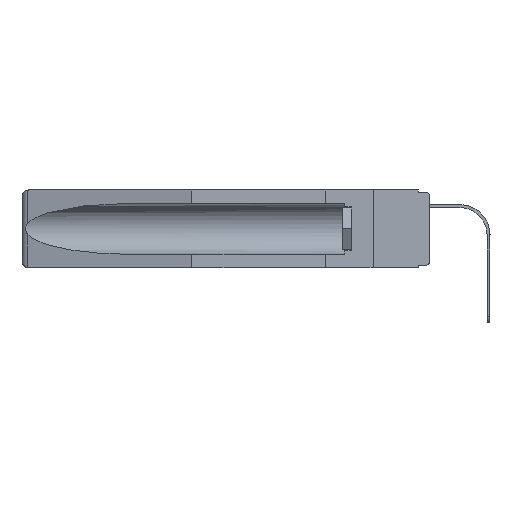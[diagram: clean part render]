
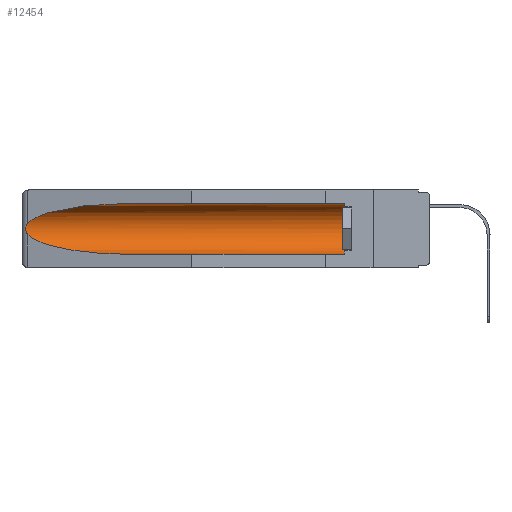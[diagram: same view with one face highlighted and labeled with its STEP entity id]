
A CAD part, left-side view. The second image highlights one B-rep face of the part: STEP entity #12454.
In plain terms, the highlighted cylindrical face has radius 2.857 mm (diameter 5.715 mm), a partial arc.
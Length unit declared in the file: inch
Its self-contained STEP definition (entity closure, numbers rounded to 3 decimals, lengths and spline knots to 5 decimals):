
#162 = VERTEX_POINT ( 'NONE', #4056 ) ;
#353 = EDGE_CURVE ( 'NONE', #4222, #19488, #18816, .T. ) ;
#668 = AXIS2_PLACEMENT_3D ( 'NONE', #8315, #3890, #9898 ) ;
#773 = CARTESIAN_POINT ( 'NONE',  ( 0.155, 0.126, -0.284 ) ) ;
#903 = CARTESIAN_POINT ( 'NONE',  ( 0.26537, 1.52718, -0.19328 ) ) ;
#1108 = CARTESIAN_POINT ( 'NONE',  ( 0.2675, 1.53308, -0.17534 ) ) ;
#1458 = EDGE_CURVE ( 'NONE', #10126, #162, #8240, .T. ) ;
#2231 = VERTEX_POINT ( 'NONE', #773 ) ;
#2311 = ORIENTED_EDGE ( 'NONE', *, *, #6201, .T. ) ;
#2358 = VERTEX_POINT ( 'NONE', #10512 ) ;
#2476 = CARTESIAN_POINT ( 'NONE',  ( 0.2675, 1.53308, -0.16763 ) ) ;
#2750 = EDGE_CURVE ( 'NONE', #2231, #2358, #17977, .T. ) ;
#3069 = CARTESIAN_POINT ( 'NONE',  ( 0.26537, 1.52718, -0.19328 ) ) ;
#3890 = DIRECTION ( 'NONE',  ( 0., -1., 0. ) ) ;
#3952 = CARTESIAN_POINT ( 'NONE',  ( 0.26655, 1.53094, -0.18657 ) ) ;
#4056 = CARTESIAN_POINT ( 'NONE',  ( 0.26537, 1.52718, -0.14972 ) ) ;
#4217 = ORIENTED_EDGE ( 'NONE', *, *, #2750, .T. ) ;
#4222 = VERTEX_POINT ( 'NONE', #18282 ) ;
#4511 = ORIENTED_EDGE ( 'NONE', *, *, #16187, .T. ) ;
#4727 = VECTOR ( 'NONE', #15743, 39.37008 ) ;
#4735 = ORIENTED_EDGE ( 'NONE', *, *, #6380, .F. ) ;
#5443 = CARTESIAN_POINT ( 'NONE',  ( 0.2673, 1.53269, -0.17917 ) ) ;
#6201 = EDGE_CURVE ( 'NONE', #2358, #10126, #7100, .T. ) ;
#6217 = CARTESIAN_POINT ( 'NONE',  ( 0.21114, 1.30732, -0.284 ) ) ;
#6380 = EDGE_CURVE ( 'NONE', #2231, #19488, #16957, .T. ) ;
#6396 = CARTESIAN_POINT ( 'NONE',  ( 0.155, 1.07973, -0.284 ) ) ;
#6759 = CARTESIAN_POINT ( 'NONE',  ( 0.155, -0.30754, -0.284 ) ) ;
#7100 = LINE ( 'NONE', #11459, #18901 ) ;
#7210 = CARTESIAN_POINT ( 'NONE',  ( 0.25451, 1.48313, -0.09465 ) ) ;
#8240 =( BOUNDED_CURVE ( )  B_SPLINE_CURVE ( 3, ( #13439, #13055, #7210, #17969 ),
 .UNSPECIFIED., .F., .F. ) 
 B_SPLINE_CURVE_WITH_KNOTS ( ( 4, 4 ),
 ( 4.71239, 6.08839 ),
 .UNSPECIFIED. ) 
 CURVE ( )  GEOMETRIC_REPRESENTATION_ITEM ( )  RATIONAL_B_SPLINE_CURVE ( ( 1., 0.848, 0.848, 1. ) ) 
 REPRESENTATION_ITEM ( '' )  );
#8315 = CARTESIAN_POINT ( 'NONE',  ( 0.155, 0.126, -0.1715 ) ) ;
#8998 = AXIS2_PLACEMENT_3D ( 'NONE', #16879, #9081, #16790 ) ;
#9081 = DIRECTION ( 'NONE',  ( 0., 1., 0. ) ) ;
#9184 = CARTESIAN_POINT ( 'NONE',  ( 0.155, 1.07973, -0.284 ) ) ;
#9898 = DIRECTION ( 'NONE',  ( 0., 0., 1. ) ) ;
#9959 = CARTESIAN_POINT ( 'NONE',  ( 0.26537, 1.52718, -0.14972 ) ) ;
#10126 = VERTEX_POINT ( 'NONE', #19419 ) ;
#10165 = CARTESIAN_POINT ( 'NONE',  ( 0.26597, 1.5296, -0.19026 ) ) ;
#10254 = CARTESIAN_POINT ( 'NONE',  ( 0.26654, 1.53092, -0.15636 ) ) ;
#10311 = ORIENTED_EDGE ( 'NONE', *, *, #1458, .T. ) ;
#10512 = CARTESIAN_POINT ( 'NONE',  ( 0.155, 0.126, -0.059 ) ) ;
#10560 = FACE_OUTER_BOUND ( 'NONE', #13226, .T. ) ;
#11459 = CARTESIAN_POINT ( 'NONE',  ( 0.155, -0.30754, -0.059 ) ) ;
#11467 = CARTESIAN_POINT ( 'NONE',  ( 0.26597, 1.52961, -0.15275 ) ) ;
#12454 = ADVANCED_FACE ( 'NONE', ( #10560 ), #15507, .F. ) ;
#12944 = CARTESIAN_POINT ( 'NONE',  ( 0.2673, 1.5327, -0.16383 ) ) ;
#13055 = CARTESIAN_POINT ( 'NONE',  ( 0.21114, 1.30732, -0.059 ) ) ;
#13226 = EDGE_LOOP ( 'NONE', ( #10311, #4511, #15786, #4735, #4217, #2311 ) ) ;
#13439 = CARTESIAN_POINT ( 'NONE',  ( 0.155, 1.07973, -0.059 ) ) ;
#13949 = B_SPLINE_CURVE_WITH_KNOTS ( 'NONE', 3,
 ( #9959, #11467, #10254, #12944, #2476, #1108, #5443, #3952, #10165, #903 ),
 .UNSPECIFIED., .F., .F.,
 ( 4, 2, 2, 2, 4 ),
 ( 0., 0.00029, 0.00058, 0.00087, 0.00117 ),
 .UNSPECIFIED. ) ;
#15214 = CARTESIAN_POINT ( 'NONE',  ( 0.25451, 1.48313, -0.24835 ) ) ;
#15507 = CYLINDRICAL_SURFACE ( 'NONE', #8998, 0.1125 ) ;
#15743 = DIRECTION ( 'NONE',  ( 0., 1., 0. ) ) ;
#15786 = ORIENTED_EDGE ( 'NONE', *, *, #353, .T. ) ;
#16187 = EDGE_CURVE ( 'NONE', #162, #4222, #13949, .T. ) ;
#16790 = DIRECTION ( 'NONE',  ( 0., 0., 1. ) ) ;
#16879 = CARTESIAN_POINT ( 'NONE',  ( 0.155, -0.30754, -0.1715 ) ) ;
#16957 = LINE ( 'NONE', #6759, #4727 ) ;
#17969 = CARTESIAN_POINT ( 'NONE',  ( 0.26537, 1.52718, -0.14972 ) ) ;
#17977 = CIRCLE ( 'NONE', #668, 0.1125 ) ;
#18282 = CARTESIAN_POINT ( 'NONE',  ( 0.26537, 1.52718, -0.19328 ) ) ;
#18816 =( BOUNDED_CURVE ( )  B_SPLINE_CURVE ( 3, ( #3069, #15214, #6217, #9184 ),
 .UNSPECIFIED., .F., .F. ) 
 B_SPLINE_CURVE_WITH_KNOTS ( ( 4, 4 ),
 ( 0.1948, 1.5708 ),
 .UNSPECIFIED. ) 
 CURVE ( )  GEOMETRIC_REPRESENTATION_ITEM ( )  RATIONAL_B_SPLINE_CURVE ( ( 1., 0.848, 0.848, 1. ) ) 
 REPRESENTATION_ITEM ( '' )  );
#18901 = VECTOR ( 'NONE', #19140, 39.37008 ) ;
#19140 = DIRECTION ( 'NONE',  ( 0., 1., 0. ) ) ;
#19419 = CARTESIAN_POINT ( 'NONE',  ( 0.155, 1.07973, -0.059 ) ) ;
#19488 = VERTEX_POINT ( 'NONE', #6396 ) ;
